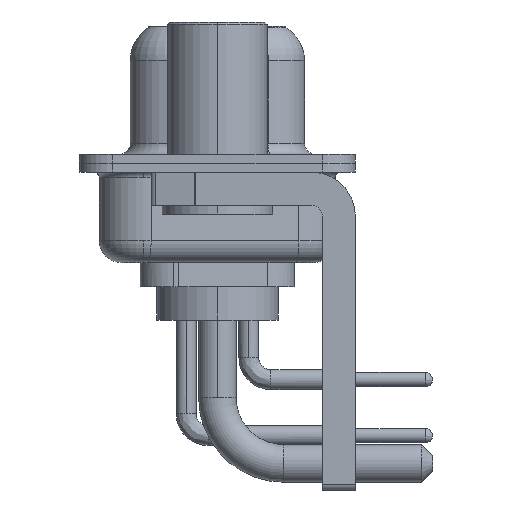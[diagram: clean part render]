
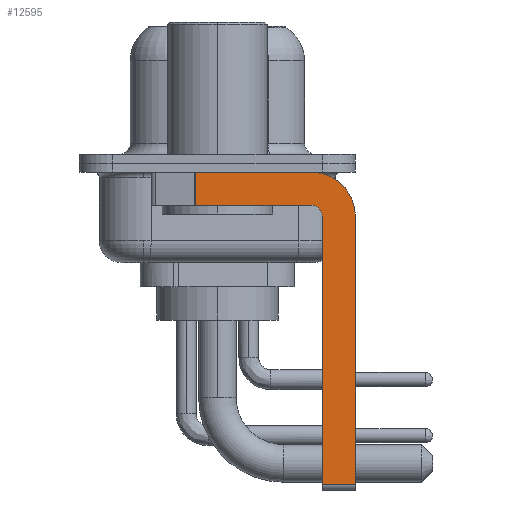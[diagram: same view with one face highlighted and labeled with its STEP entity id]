
A CAD part, left-side view. The second image highlights one B-rep face of the part: STEP entity #12595.
In plain terms, the highlighted planar face has unit normal (-1, 0, 0).
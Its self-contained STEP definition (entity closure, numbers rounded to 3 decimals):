
#88 = VECTOR ( 'NONE', #3737, 1000. ) ;
#279 = ORIENTED_EDGE ( 'NONE', *, *, #5667, .F. ) ;
#821 = CARTESIAN_POINT ( 'NONE',  ( -2.9, -4.25, -2.4 ) ) ;
#1801 = CARTESIAN_POINT ( 'NONE',  ( -2.9, 0.978, -1.9 ) ) ;
#1832 = LINE ( 'NONE', #12554, #2887 ) ;
#2577 = VERTEX_POINT ( 'NONE', #14820 ) ;
#2770 = VERTEX_POINT ( 'NONE', #16684 ) ;
#2887 = VECTOR ( 'NONE', #10892, 1000. ) ;
#3247 = CARTESIAN_POINT ( 'NONE',  ( -2.9, -4.25, -2.4 ) ) ;
#3419 = EDGE_CURVE ( 'NONE', #18172, #2577, #16380, .T. ) ;
#3430 = DIRECTION ( 'NONE',  ( 1., 0., 0. ) ) ;
#3440 = CARTESIAN_POINT ( 'NONE',  ( -2.9, -4.75, -14.8 ) ) ;
#3463 = DIRECTION ( 'NONE',  ( 0., 0., 1. ) ) ;
#3737 = DIRECTION ( 'NONE',  ( 0., -1., 0. ) ) ;
#3889 = LINE ( 'NONE', #14319, #13939 ) ;
#4078 = ORIENTED_EDGE ( 'NONE', *, *, #9161, .F. ) ;
#4158 = VERTEX_POINT ( 'NONE', #13598 ) ;
#4299 = VERTEX_POINT ( 'NONE', #1801 ) ;
#4423 = LINE ( 'NONE', #3440, #10700 ) ;
#4839 = ORIENTED_EDGE ( 'NONE', *, *, #3419, .F. ) ;
#5211 = CARTESIAN_POINT ( 'NONE',  ( -2.9, 3., -0.4 ) ) ;
#5227 = DIRECTION ( 'NONE',  ( 1., 0., 0. ) ) ;
#5265 = DIRECTION ( 'NONE',  ( 0., -1., 0. ) ) ;
#5587 = CARTESIAN_POINT ( 'NONE',  ( -2.9, -4.75, -2.4 ) ) ;
#5667 = EDGE_CURVE ( 'NONE', #8467, #12816, #18808, .T. ) ;
#6025 = AXIS2_PLACEMENT_3D ( 'NONE', #3247, #3430, #15230 ) ;
#6172 = EDGE_CURVE ( 'NONE', #12816, #4299, #14425, .T. ) ;
#6381 = VECTOR ( 'NONE', #16477, 1000. ) ;
#6525 = CARTESIAN_POINT ( 'NONE',  ( -2.9, -4.25, -2.4 ) ) ;
#6694 = DIRECTION ( 'NONE',  ( 0., 1., 0. ) ) ;
#6964 = CARTESIAN_POINT ( 'NONE',  ( -2.9, -4.25, -1.9 ) ) ;
#7258 = EDGE_CURVE ( 'NONE', #2770, #8467, #4423, .T. ) ;
#8003 = ORIENTED_EDGE ( 'NONE', *, *, #8328, .F. ) ;
#8217 = CARTESIAN_POINT ( 'NONE',  ( -2.9, -4.25, -0.4 ) ) ;
#8328 = EDGE_CURVE ( 'NONE', #4158, #18172, #18684, .T. ) ;
#8467 = VERTEX_POINT ( 'NONE', #5587 ) ;
#8898 = ORIENTED_EDGE ( 'NONE', *, *, #7258, .F. ) ;
#9029 = CARTESIAN_POINT ( 'NONE',  ( -2.9, -6.25, -14.55 ) ) ;
#9161 = EDGE_CURVE ( 'NONE', #2577, #11097, #19420, .T. ) ;
#9595 = AXIS2_PLACEMENT_3D ( 'NONE', #821, #5227, #11251 ) ;
#10700 = VECTOR ( 'NONE', #18481, 1000. ) ;
#10892 = DIRECTION ( 'NONE',  ( 0., 0., -1. ) ) ;
#11097 = VERTEX_POINT ( 'NONE', #9029 ) ;
#11102 = ORIENTED_EDGE ( 'NONE', *, *, #11358, .T. ) ;
#11251 = DIRECTION ( 'NONE',  ( 0., 0., -1. ) ) ;
#11358 = EDGE_CURVE ( 'NONE', #2770, #11097, #3889, .T. ) ;
#11939 = VECTOR ( 'NONE', #6694, 1000. ) ;
#12554 = CARTESIAN_POINT ( 'NONE',  ( -2.9, 0.978, -1.9 ) ) ;
#12595 = ADVANCED_FACE ( 'NONE', ( #12711 ), #18697, .F. ) ;
#12711 = FACE_OUTER_BOUND ( 'NONE', #14491, .T. ) ;
#12816 = VERTEX_POINT ( 'NONE', #16607 ) ;
#13437 = CARTESIAN_POINT ( 'NONE',  ( -2.9, -6.25, -2.4 ) ) ;
#13598 = CARTESIAN_POINT ( 'NONE',  ( -2.9, 0.978, -0.4 ) ) ;
#13939 = VECTOR ( 'NONE', #5265, 1000. ) ;
#14319 = CARTESIAN_POINT ( 'NONE',  ( -2.9, -4.25, -14.55 ) ) ;
#14425 = LINE ( 'NONE', #6964, #11939 ) ;
#14491 = EDGE_LOOP ( 'NONE', ( #8003, #16537, #16075, #279, #8898, #11102, #4078, #4839 ) ) ;
#14820 = CARTESIAN_POINT ( 'NONE',  ( -2.9, -6.25, -2.4 ) ) ;
#15230 = DIRECTION ( 'NONE',  ( 0., 0., -1. ) ) ;
#16075 = ORIENTED_EDGE ( 'NONE', *, *, #6172, .F. ) ;
#16380 = CIRCLE ( 'NONE', #6025, 2. ) ;
#16477 = DIRECTION ( 'NONE',  ( 0., 0., -1. ) ) ;
#16537 = ORIENTED_EDGE ( 'NONE', *, *, #18044, .T. ) ;
#16607 = CARTESIAN_POINT ( 'NONE',  ( -2.9, -4.25, -1.9 ) ) ;
#16609 = AXIS2_PLACEMENT_3D ( 'NONE', #6525, #16929, #3463 ) ;
#16684 = CARTESIAN_POINT ( 'NONE',  ( -2.9, -4.75, -14.55 ) ) ;
#16929 = DIRECTION ( 'NONE',  ( -1., 0., 0. ) ) ;
#18044 = EDGE_CURVE ( 'NONE', #4158, #4299, #1832, .T. ) ;
#18172 = VERTEX_POINT ( 'NONE', #8217 ) ;
#18481 = DIRECTION ( 'NONE',  ( 0., 0., 1. ) ) ;
#18684 = LINE ( 'NONE', #5211, #88 ) ;
#18697 = PLANE ( 'NONE',  #9595 ) ;
#18808 = CIRCLE ( 'NONE', #16609, 0.5 ) ;
#19420 = LINE ( 'NONE', #13437, #6381 ) ;
